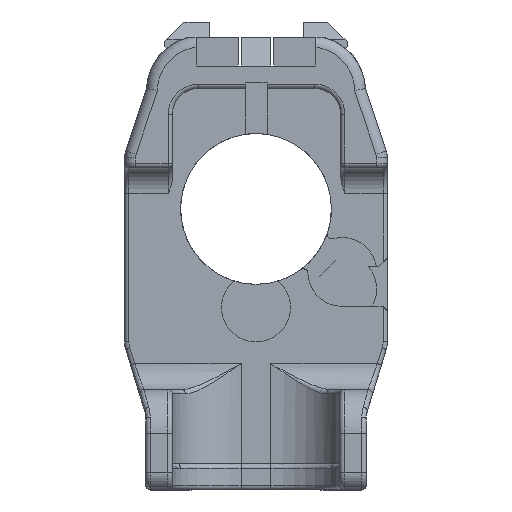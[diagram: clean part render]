
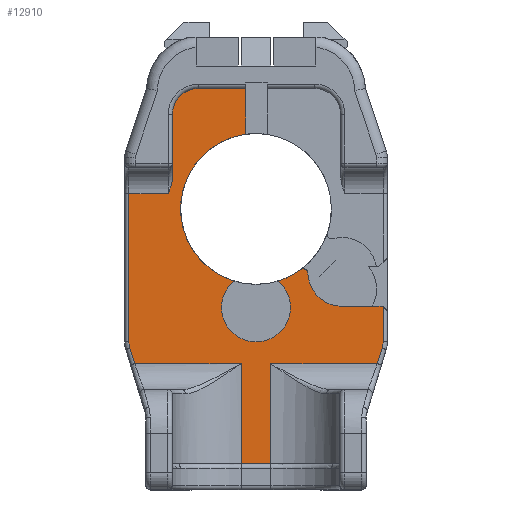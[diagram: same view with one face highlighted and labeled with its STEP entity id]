
A CAD part, front view. The second image highlights one B-rep face of the part: STEP entity #12910.
In plain terms, the highlighted planar face has unit normal (0, -1, 0).
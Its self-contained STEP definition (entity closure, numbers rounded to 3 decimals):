
#86=B_SPLINE_CURVE_WITH_KNOTS('',3,(#19895,#19896,#19897,#19898),
 .UNSPECIFIED.,.F.,.F.,(4,4),(0.382,0.56),
 .UNSPECIFIED.);
#363=CIRCLE('',#13577,8.75);
#365=CIRCLE('',#13579,8.75);
#375=CIRCLE('',#13686,3.);
#377=CIRCLE('',#13689,2.5);
#378=CIRCLE('',#13690,2.5);
#379=CIRCLE('',#13691,4.);
#380=CIRCLE('',#13692,0.5);
#381=CIRCLE('',#13693,4.);
#811=FACE_OUTER_BOUND('',#1547,.T.);
#1547=EDGE_LOOP('',(#9594,#9595,#9596,#9597,#9598,#9599,#9600,#9601,#9602,
#9603,#9604,#9605,#9606,#9607,#9608,#9609,#9610,#9611,#9612,#9613,#9614,
#9615,#9616));
#2747=LINE('',#19868,#4305);
#2749=LINE('',#19872,#4307);
#2755=LINE('',#19893,#4313);
#2756=LINE('',#19900,#4314);
#2757=LINE('',#19902,#4315);
#2758=LINE('',#19906,#4316);
#2759=LINE('',#19908,#4317);
#2760=LINE('',#19910,#4318);
#2761=LINE('',#19912,#4319);
#2762=LINE('',#19914,#4320);
#2763=LINE('',#19916,#4321);
#2764=LINE('',#19918,#4322);
#2765=LINE('',#19922,#4323);
#2766=LINE('',#19924,#4324);
#4305=VECTOR('',#15600,10.);
#4307=VECTOR('',#15604,10.);
#4313=VECTOR('',#15624,10.);
#4314=VECTOR('',#15625,10.);
#4315=VECTOR('',#15626,10.);
#4316=VECTOR('',#15629,10.);
#4317=VECTOR('',#15630,10.);
#4318=VECTOR('',#15631,10.);
#4319=VECTOR('',#15632,10.);
#4320=VECTOR('',#15633,10.);
#4321=VECTOR('',#15634,10.);
#4322=VECTOR('',#15635,10.);
#4323=VECTOR('',#15638,10.);
#4324=VECTOR('',#15639,10.);
#5518=VERTEX_POINT('',#19225);
#5519=VERTEX_POINT('',#19227);
#5522=VERTEX_POINT('',#19233);
#5523=VERTEX_POINT('',#19235);
#5683=VERTEX_POINT('',#19866);
#5684=VERTEX_POINT('',#19871);
#5690=VERTEX_POINT('',#19886);
#5692=VERTEX_POINT('',#19892);
#5693=VERTEX_POINT('',#19894);
#5694=VERTEX_POINT('',#19899);
#5695=VERTEX_POINT('',#19901);
#5696=VERTEX_POINT('',#19903);
#5697=VERTEX_POINT('',#19905);
#5698=VERTEX_POINT('',#19907);
#5699=VERTEX_POINT('',#19909);
#5700=VERTEX_POINT('',#19911);
#5701=VERTEX_POINT('',#19913);
#5702=VERTEX_POINT('',#19915);
#5703=VERTEX_POINT('',#19917);
#5704=VERTEX_POINT('',#19919);
#5705=VERTEX_POINT('',#19921);
#5706=VERTEX_POINT('',#19923);
#5707=VERTEX_POINT('',#19925);
#6841=EDGE_CURVE('',#5519,#5518,#363,.T.);
#6845=EDGE_CURVE('',#5523,#5522,#365,.T.);
#7101=EDGE_CURVE('',#5683,#5518,#2747,.T.);
#7103=EDGE_CURVE('',#5683,#5684,#2749,.T.);
#7110=EDGE_CURVE('',#5684,#5690,#375,.T.);
#7113=EDGE_CURVE('',#5690,#5692,#2755,.T.);
#7114=EDGE_CURVE('',#5693,#5692,#86,.F.);
#7115=EDGE_CURVE('',#5694,#5693,#2756,.T.);
#7116=EDGE_CURVE('',#5695,#5694,#2757,.T.);
#7117=EDGE_CURVE('',#5696,#5695,#377,.T.);
#7118=EDGE_CURVE('',#5697,#5696,#2758,.T.);
#7119=EDGE_CURVE('',#5697,#5698,#2759,.T.);
#7120=EDGE_CURVE('',#5699,#5698,#2760,.T.);
#7121=EDGE_CURVE('',#5699,#5700,#2761,.T.);
#7122=EDGE_CURVE('',#5701,#5700,#2762,.T.);
#7123=EDGE_CURVE('',#5701,#5702,#2763,.T.);
#7124=EDGE_CURVE('',#5703,#5702,#2764,.T.);
#7125=EDGE_CURVE('',#5704,#5703,#378,.T.);
#7126=EDGE_CURVE('',#5705,#5704,#2765,.T.);
#7127=EDGE_CURVE('',#5706,#5705,#2766,.T.);
#7128=EDGE_CURVE('',#5706,#5707,#379,.T.);
#7129=EDGE_CURVE('',#5523,#5707,#380,.T.);
#7130=EDGE_CURVE('',#5522,#5519,#381,.T.);
#9594=ORIENTED_EDGE('',*,*,#7110,.T.);
#9595=ORIENTED_EDGE('',*,*,#7113,.T.);
#9596=ORIENTED_EDGE('',*,*,#7114,.F.);
#9597=ORIENTED_EDGE('',*,*,#7115,.F.);
#9598=ORIENTED_EDGE('',*,*,#7116,.F.);
#9599=ORIENTED_EDGE('',*,*,#7117,.F.);
#9600=ORIENTED_EDGE('',*,*,#7118,.F.);
#9601=ORIENTED_EDGE('',*,*,#7119,.T.);
#9602=ORIENTED_EDGE('',*,*,#7120,.F.);
#9603=ORIENTED_EDGE('',*,*,#7121,.T.);
#9604=ORIENTED_EDGE('',*,*,#7122,.F.);
#9605=ORIENTED_EDGE('',*,*,#7123,.T.);
#9606=ORIENTED_EDGE('',*,*,#7124,.F.);
#9607=ORIENTED_EDGE('',*,*,#7125,.F.);
#9608=ORIENTED_EDGE('',*,*,#7126,.F.);
#9609=ORIENTED_EDGE('',*,*,#7127,.F.);
#9610=ORIENTED_EDGE('',*,*,#7128,.T.);
#9611=ORIENTED_EDGE('',*,*,#7129,.F.);
#9612=ORIENTED_EDGE('',*,*,#6845,.T.);
#9613=ORIENTED_EDGE('',*,*,#7130,.T.);
#9614=ORIENTED_EDGE('',*,*,#6841,.T.);
#9615=ORIENTED_EDGE('',*,*,#7101,.F.);
#9616=ORIENTED_EDGE('',*,*,#7103,.T.);
#12357=PLANE('',#13688);
#12910=ADVANCED_FACE('',(#811),#12357,.T.);
#13577=AXIS2_PLACEMENT_3D('',#19228,#15152,#15153);
#13579=AXIS2_PLACEMENT_3D('',#19236,#15158,#15159);
#13686=AXIS2_PLACEMENT_3D('',#19887,#15617,#15618);
#13688=AXIS2_PLACEMENT_3D('',#19891,#15622,#15623);
#13689=AXIS2_PLACEMENT_3D('',#19904,#15627,#15628);
#13690=AXIS2_PLACEMENT_3D('',#19920,#15636,#15637);
#13691=AXIS2_PLACEMENT_3D('',#19926,#15640,#15641);
#13692=AXIS2_PLACEMENT_3D('',#19927,#15642,#15643);
#13693=AXIS2_PLACEMENT_3D('',#19928,#15644,#15645);
#15152=DIRECTION('center_axis',(0.,1.,0.));
#15153=DIRECTION('ref_axis',(-1.,0.,0.));
#15158=DIRECTION('center_axis',(0.,1.,0.));
#15159=DIRECTION('ref_axis',(-1.,0.,0.));
#15600=DIRECTION('',(0.,0.,-1.));
#15604=DIRECTION('',(-1.,0.,0.));
#15617=DIRECTION('center_axis',(0.,-1.,0.));
#15618=DIRECTION('ref_axis',(-1.,0.,0.));
#15622=DIRECTION('center_axis',(0.,-1.,0.));
#15623=DIRECTION('ref_axis',(0.,0.,-1.));
#15624=DIRECTION('',(0.,0.,-1.));
#15625=DIRECTION('',(1.,0.,0.));
#15626=DIRECTION('',(0.,0.,1.));
#15627=DIRECTION('center_axis',(0.,1.,0.));
#15628=DIRECTION('ref_axis',(-0.989,0.,-0.149));
#15629=DIRECTION('',(-0.294,0.,0.956));
#15630=DIRECTION('',(1.,0.,0.));
#15631=DIRECTION('',(0.,0.,1.));
#15632=DIRECTION('',(1.,0.,0.));
#15633=DIRECTION('',(0.,0.,-1.));
#15634=DIRECTION('',(1.,0.,0.));
#15635=DIRECTION('',(-0.294,0.,-0.956));
#15636=DIRECTION('center_axis',(0.,1.,0.));
#15637=DIRECTION('ref_axis',(0.989,0.,-0.149));
#15638=DIRECTION('',(0.,0.,-1.));
#15639=DIRECTION('',(1.,0.,0.));
#15640=DIRECTION('center_axis',(0.,1.,0.));
#15641=DIRECTION('ref_axis',(-0.751,0.,0.66));
#15642=DIRECTION('center_axis',(0.,1.,0.));
#15643=DIRECTION('ref_axis',(0.437,0.,0.9));
#15644=DIRECTION('center_axis',(0.,1.,0.));
#15645=DIRECTION('ref_axis',(1.,0.,0.));
#19225=CARTESIAN_POINT('',(-1.212,65.024,-94.904));
#19227=CARTESIAN_POINT('',(-2.569,65.024,-111.934));
#19228=CARTESIAN_POINT('Origin',(0.,65.024,-103.57));
#19233=CARTESIAN_POINT('',(2.569,65.024,-111.934));
#19235=CARTESIAN_POINT('',(5.205,65.024,-110.604));
#19236=CARTESIAN_POINT('Origin',(0.,65.024,-103.57));
#19866=CARTESIAN_POINT('',(-1.212,65.024,-89.606));
#19868=CARTESIAN_POINT('',(-1.212,65.024,-101.281));
#19871=CARTESIAN_POINT('',(-6.692,65.024,-89.606));
#19872=CARTESIAN_POINT('',(-12.701,65.024,-89.606));
#19886=CARTESIAN_POINT('',(-9.692,65.024,-92.606));
#19887=CARTESIAN_POINT('Origin',(-6.692,65.024,-92.606));
#19891=CARTESIAN_POINT('Origin',(-12.7,65.024,-107.382));
#19892=CARTESIAN_POINT('',(-9.692,65.024,-100.002));
#19893=CARTESIAN_POINT('',(-9.692,65.024,-103.093));
#19894=CARTESIAN_POINT('',(-10.192,65.024,-101.805));
#19895=CARTESIAN_POINT('Ctrl Pts',(-9.692,65.024,-100.002));
#19896=CARTESIAN_POINT('Ctrl Pts',(-9.692,65.024,-100.597));
#19897=CARTESIAN_POINT('Ctrl Pts',(-9.968,65.024,-101.255));
#19898=CARTESIAN_POINT('Ctrl Pts',(-10.192,65.024,-101.805));
#19899=CARTESIAN_POINT('',(-14.74,65.024,-101.805));
#19900=CARTESIAN_POINT('',(-13.97,65.024,-101.805));
#19901=CARTESIAN_POINT('',(-14.74,65.024,-118.994));
#19902=CARTESIAN_POINT('',(-14.74,65.024,-105.95));
#19903=CARTESIAN_POINT('',(-14.629,65.024,-119.729));
#19904=CARTESIAN_POINT('Origin',(-12.24,65.024,-118.994));
#19905=CARTESIAN_POINT('',(-14.077,65.024,-121.525));
#19906=CARTESIAN_POINT('',(-15.078,65.024,-118.272));
#19907=CARTESIAN_POINT('',(-1.723,65.024,-121.525));
#19908=CARTESIAN_POINT('',(-10.795,65.024,-121.525));
#19909=CARTESIAN_POINT('',(-1.723,65.024,-133.145));
#19910=CARTESIAN_POINT('',(-1.723,65.024,-123.763));
#19911=CARTESIAN_POINT('',(1.723,65.024,-133.145));
#19912=CARTESIAN_POINT('',(-6.35,65.024,-133.145));
#19913=CARTESIAN_POINT('',(1.723,65.024,-121.525));
#19914=CARTESIAN_POINT('',(1.723,65.024,-116.066));
#19915=CARTESIAN_POINT('',(14.077,65.024,-121.525));
#19916=CARTESIAN_POINT('',(1.27,65.024,-121.525));
#19917=CARTESIAN_POINT('',(14.629,65.024,-119.729));
#19918=CARTESIAN_POINT('',(16.519,65.024,-113.587));
#19919=CARTESIAN_POINT('',(14.74,65.024,-118.994));
#19920=CARTESIAN_POINT('Origin',(12.24,65.024,-118.994));
#19921=CARTESIAN_POINT('',(14.74,65.024,-114.871));
#19922=CARTESIAN_POINT('',(14.74,65.024,-105.945));
#19923=CARTESIAN_POINT('',(9.906,65.024,-114.871));
#19924=CARTESIAN_POINT('',(9.953,65.024,-114.871));
#19925=CARTESIAN_POINT('',(6.002,65.024,-110.991));
#19926=CARTESIAN_POINT('Origin',(10.,65.024,-110.872));
#19927=CARTESIAN_POINT('Origin',(5.502,65.024,-111.006));
#19928=CARTESIAN_POINT('Origin',(0.,65.024,-115.));
